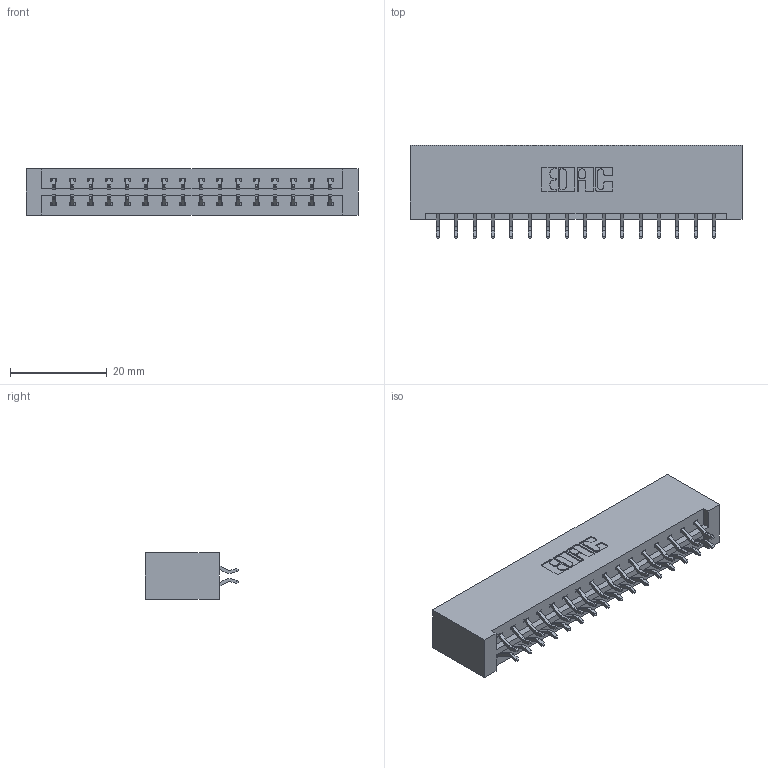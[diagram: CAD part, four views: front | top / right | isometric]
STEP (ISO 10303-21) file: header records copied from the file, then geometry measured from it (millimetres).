
FILE_DESCRIPTION (( 'STEP AP203' ), '1' );
FILE_NAME ('379-032-556-201.STEP', '2020-09-30T17:26:30', ( '' ), ( '' ), 'SwSTEP 2.0', 'SolidWorks 2020', '' );
FILE_SCHEMA (( 'CONFIG_CONTROL_DESIGN' ));
Length unit declared in the file: inch
Products named in the file (3): 379-032-556-201; 379 Part_Lugless; 345-292-001_556 Tail
Assembly tree (33 placements, depth 2):
  379-032-556-201
    379 Part_Lugless
    345-292-001_556 Tail  x32
Bounding box: 68.58 x 19.24 x 9.53 mm (x, y, z)
Volume: 7719.1 mm3; surface area: 8437.6 mm2
Topology: 33 solids, 33 shells, 1962 faces, 5823 edges, 3838 vertices
Faces by surface type: plane 1346, cylinder 616
Entity records: 13599 total; most frequent: CARTESIAN_POINT 2298, ORIENTED_EDGE 2222, DIRECTION 1991, EDGE_CURVE 1111, LINE 983, VECTOR 983, VERTEX_POINT 738, AXIS2_PLACEMENT_3D 504
